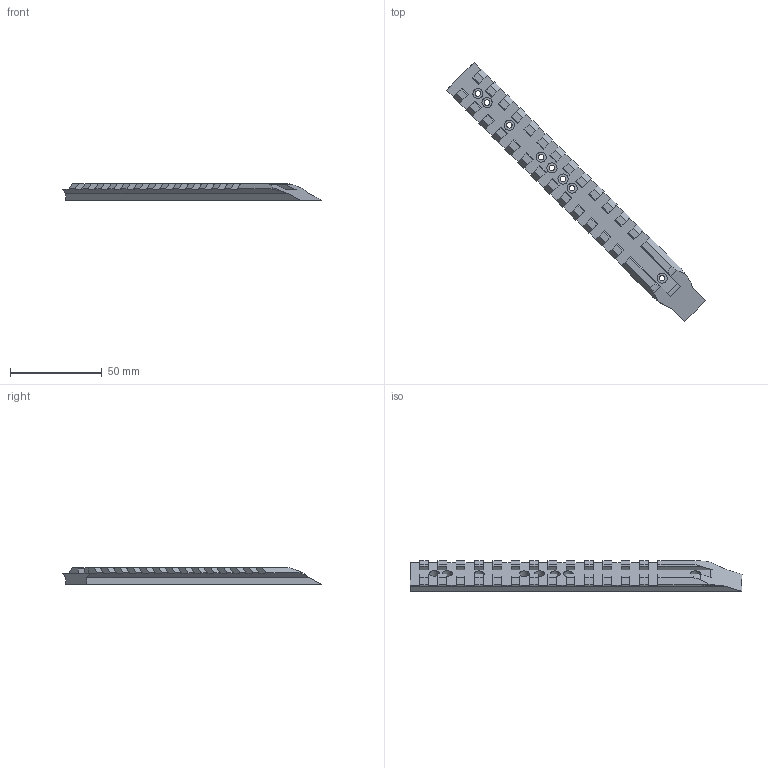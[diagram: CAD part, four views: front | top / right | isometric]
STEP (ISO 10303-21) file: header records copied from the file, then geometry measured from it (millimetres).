
FILE_DESCRIPTION(/* description */ (''),/* implementation_level */ '2;1');
FILE_NAME(/* name */ 'Top Rail Front Half.step',/* time_stamp */ '2022-05-11T21:22:19-06:00',/* author */ (''),/* organization */ (''),/* preprocessor_version */ 'ST-DEVELOPER v18.1',/* originating_system */ 'Autodesk Translation Framework v10.10.0.1391',/* authorisation */ '');
FILE_SCHEMA (('AUTOMOTIVE_DESIGN { 1 0 10303 214 3 1 1 }'));
Length unit declared in the file: millimetre
Products named in the file (1): Top Rail tall front (1)
Bounding box: 141.25 x 141.25 x 9 mm (x, y, z)
Volume: 19925.7 mm3; surface area: 11545.4 mm2
Topology: 1 solids, 1 shells, 209 faces, 589 edges, 392 vertices
Faces by surface type: plane 186, cylinder 23
Full cylindrical faces by diameter (mm): 3 x9, 5 x1, 5.5 x8
Entity records: 6729 total; most frequent: CARTESIAN_POINT 1191, ORIENTED_EDGE 1178, DIRECTION 1059, EDGE_CURVE 589, LINE 539, VECTOR 539, VERTEX_POINT 392, AXIS2_PLACEMENT_3D 260
